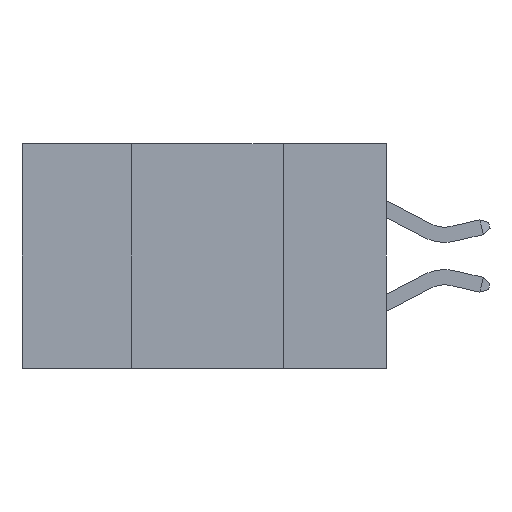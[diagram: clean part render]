
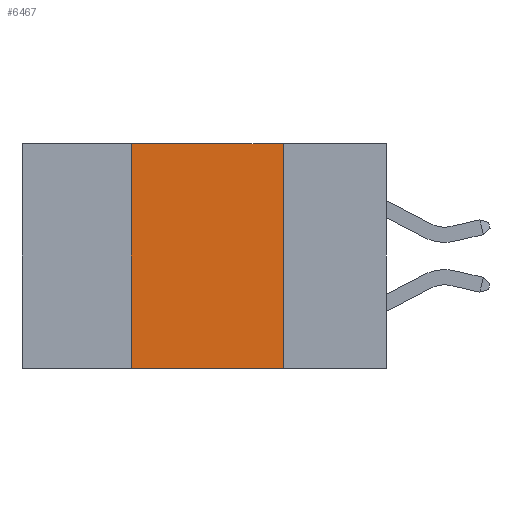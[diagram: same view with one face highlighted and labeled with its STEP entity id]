
A CAD part, left-side view. The second image highlights one B-rep face of the part: STEP entity #6467.
In plain terms, the highlighted planar face has unit normal (-1, 0, 0).
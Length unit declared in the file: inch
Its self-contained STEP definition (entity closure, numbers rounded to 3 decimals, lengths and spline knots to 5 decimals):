
#532 = CARTESIAN_POINT ( 'NONE',  ( 0., 0.42, -0.37 ) ) ;
#773 = CARTESIAN_POINT ( 'NONE',  ( 0., 0.42, 0. ) ) ;
#919 = DIRECTION ( 'NONE',  ( 0., -1., 0. ) ) ;
#1115 = CARTESIAN_POINT ( 'NONE',  ( 0., 0.6, 0. ) ) ;
#1212 = VERTEX_POINT ( 'NONE', #6819 ) ;
#1305 = AXIS2_PLACEMENT_3D ( 'NONE', #7211, #8109, #3853 ) ;
#1355 = LINE ( 'NONE', #1115, #9643 ) ;
#1591 = EDGE_LOOP ( 'NONE', ( #2009, #8435, #7730, #2990 ) ) ;
#1873 = EDGE_CURVE ( 'NONE', #1212, #10147, #9472, .T. ) ;
#2009 = ORIENTED_EDGE ( 'NONE', *, *, #8928, .F. ) ;
#2686 = CARTESIAN_POINT ( 'NONE',  ( 0., 0.17, -0.37 ) ) ;
#2780 = CARTESIAN_POINT ( 'NONE',  ( 0., 0.17, 0. ) ) ;
#2990 = ORIENTED_EDGE ( 'NONE', *, *, #1873, .T. ) ;
#3448 = CARTESIAN_POINT ( 'NONE',  ( 0., 0.6, -0.37 ) ) ;
#3853 = DIRECTION ( 'NONE',  ( 0., 0., -1. ) ) ;
#3955 = LINE ( 'NONE', #532, #6360 ) ;
#4544 = DIRECTION ( 'NONE',  ( 0., -1., 0. ) ) ;
#4614 = VECTOR ( 'NONE', #10600, 39.37008 ) ;
#4736 = FACE_OUTER_BOUND ( 'NONE', #1591, .T. ) ;
#4793 = PLANE ( 'NONE',  #1305 ) ;
#6360 = VECTOR ( 'NONE', #10660, 39.37008 ) ;
#6467 = ADVANCED_FACE ( 'NONE', ( #4736 ), #4793, .F. ) ;
#6819 = CARTESIAN_POINT ( 'NONE',  ( 0., 0.42, -0.37 ) ) ;
#7211 = CARTESIAN_POINT ( 'NONE',  ( 0., 0.6, 0. ) ) ;
#7423 = VERTEX_POINT ( 'NONE', #773 ) ;
#7522 = CARTESIAN_POINT ( 'NONE',  ( 0., 0.17, -0.37 ) ) ;
#7730 = ORIENTED_EDGE ( 'NONE', *, *, #7791, .F. ) ;
#7791 = EDGE_CURVE ( 'NONE', #1212, #7423, #3955, .T. ) ;
#7853 = VECTOR ( 'NONE', #919, 39.37008 ) ;
#8021 = VERTEX_POINT ( 'NONE', #2780 ) ;
#8109 = DIRECTION ( 'NONE',  ( 1., 0., 0. ) ) ;
#8435 = ORIENTED_EDGE ( 'NONE', *, *, #8685, .F. ) ;
#8685 = EDGE_CURVE ( 'NONE', #7423, #8021, #1355, .T. ) ;
#8928 = EDGE_CURVE ( 'NONE', #8021, #10147, #10384, .T. ) ;
#9472 = LINE ( 'NONE', #3448, #7853 ) ;
#9643 = VECTOR ( 'NONE', #4544, 39.37008 ) ;
#10147 = VERTEX_POINT ( 'NONE', #7522 ) ;
#10384 = LINE ( 'NONE', #2686, #4614 ) ;
#10600 = DIRECTION ( 'NONE',  ( 0., 0., -1. ) ) ;
#10660 = DIRECTION ( 'NONE',  ( 0., 0., 1. ) ) ;
